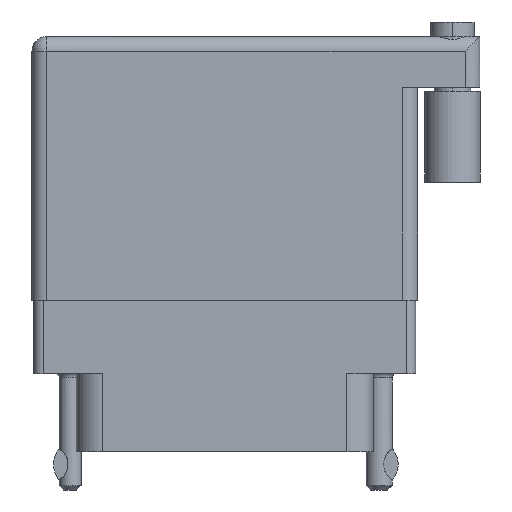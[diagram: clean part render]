
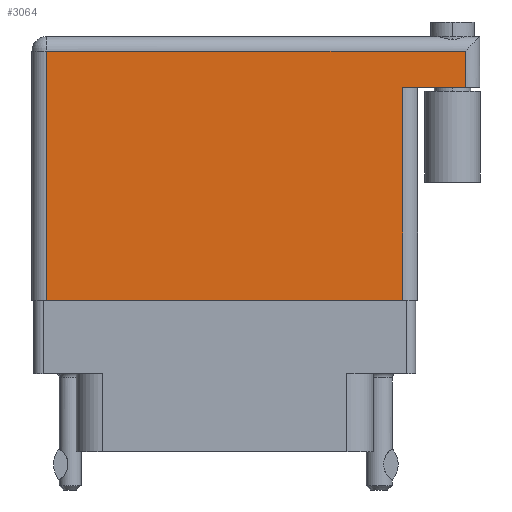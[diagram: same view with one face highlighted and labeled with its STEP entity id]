
A CAD part, front view. The second image highlights one B-rep face of the part: STEP entity #3064.
In plain terms, the highlighted face is planar.
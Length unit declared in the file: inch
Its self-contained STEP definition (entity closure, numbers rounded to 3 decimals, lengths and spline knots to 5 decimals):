
#258 = DIRECTION ( 'NONE',  ( -1., 0., 0. ) ) ;
#670 = EDGE_CURVE ( 'NONE', #27080, #21208, #31366, .T. ) ;
#1006 = ORIENTED_EDGE ( 'NONE', *, *, #4746, .F. ) ;
#1188 = DIRECTION ( 'NONE',  ( 0., 1., 0. ) ) ;
#1465 = CARTESIAN_POINT ( 'NONE',  ( 1.275, 0.731, 0. ) ) ;
#1528 = VERTEX_POINT ( 'NONE', #18580 ) ;
#3013 = LINE ( 'NONE', #14241, #13957 ) ;
#3064 = ADVANCED_FACE ( 'NONE', ( #22866 ), #33910, .F. ) ;
#3598 = VECTOR ( 'NONE', #20691, 39.37008 ) ;
#4746 = EDGE_CURVE ( 'NONE', #9153, #1528, #7953, .T. ) ;
#5846 = EDGE_CURVE ( 'NONE', #21208, #1528, #31854, .T. ) ;
#7746 = EDGE_CURVE ( 'NONE', #24611, #27080, #3013, .T. ) ;
#7953 = LINE ( 'NONE', #18998, #23412 ) ;
#8746 = DIRECTION ( 'NONE',  ( 0., 0., -1. ) ) ;
#8852 = CARTESIAN_POINT ( 'NONE',  ( 0.05, 0.856, 0. ) ) ;
#9110 = CARTESIAN_POINT ( 'NONE',  ( 0., 0.906, 0. ) ) ;
#9153 = VERTEX_POINT ( 'NONE', #26653 ) ;
#11836 = VECTOR ( 'NONE', #1188, 39.37008 ) ;
#12308 = EDGE_CURVE ( 'NONE', #30408, #24611, #19021, .T. ) ;
#13046 = DIRECTION ( 'NONE',  ( 0., 1., 0. ) ) ;
#13957 = VECTOR ( 'NONE', #33417, 39.37008 ) ;
#14241 = CARTESIAN_POINT ( 'NONE',  ( 0.05, 0., 0. ) ) ;
#17090 = EDGE_LOOP ( 'NONE', ( #31367, #17917, #1006, #24808, #35227, #31165 ) ) ;
#17650 = CARTESIAN_POINT ( 'NONE',  ( 0., 0., 0. ) ) ;
#17917 = ORIENTED_EDGE ( 'NONE', *, *, #5846, .T. ) ;
#18580 = CARTESIAN_POINT ( 'NONE',  ( 1.275, 0.731, 0. ) ) ;
#18998 = CARTESIAN_POINT ( 'NONE',  ( 1.539, 0.731, 0. ) ) ;
#19021 = LINE ( 'NONE', #19378, #25669 ) ;
#19378 = CARTESIAN_POINT ( 'NONE',  ( 0., 0.856, 0. ) ) ;
#20565 = VECTOR ( 'NONE', #13046, 39.37008 ) ;
#20691 = DIRECTION ( 'NONE',  ( 1., 0., 0. ) ) ;
#21208 = VERTEX_POINT ( 'NONE', #22982 ) ;
#22262 = CARTESIAN_POINT ( 'NONE',  ( 0.05, 0., 0. ) ) ;
#22857 = CARTESIAN_POINT ( 'NONE',  ( 1.489, 0.856, 0. ) ) ;
#22866 = FACE_OUTER_BOUND ( 'NONE', #17090, .T. ) ;
#22982 = CARTESIAN_POINT ( 'NONE',  ( 1.275, 0., 0. ) ) ;
#23412 = VECTOR ( 'NONE', #26939, 39.37008 ) ;
#24611 = VERTEX_POINT ( 'NONE', #8852 ) ;
#24808 = ORIENTED_EDGE ( 'NONE', *, *, #29060, .T. ) ;
#25422 = CARTESIAN_POINT ( 'NONE',  ( 1.489, 0.906, 0. ) ) ;
#25669 = VECTOR ( 'NONE', #27666, 39.37008 ) ;
#26653 = CARTESIAN_POINT ( 'NONE',  ( 1.489, 0.731, 0. ) ) ;
#26939 = DIRECTION ( 'NONE',  ( -1., 0., 0. ) ) ;
#27080 = VERTEX_POINT ( 'NONE', #22262 ) ;
#27666 = DIRECTION ( 'NONE',  ( -1., 0., 0. ) ) ;
#28705 = LINE ( 'NONE', #25422, #11836 ) ;
#29060 = EDGE_CURVE ( 'NONE', #9153, #30408, #28705, .T. ) ;
#30408 = VERTEX_POINT ( 'NONE', #22857 ) ;
#31165 = ORIENTED_EDGE ( 'NONE', *, *, #7746, .T. ) ;
#31366 = LINE ( 'NONE', #17650, #3598 ) ;
#31367 = ORIENTED_EDGE ( 'NONE', *, *, #670, .T. ) ;
#31854 = LINE ( 'NONE', #1465, #20565 ) ;
#33417 = DIRECTION ( 'NONE',  ( 0., -1., 0. ) ) ;
#33910 = PLANE ( 'NONE',  #34505 ) ;
#34505 = AXIS2_PLACEMENT_3D ( 'NONE', #9110, #8746, #258 ) ;
#35227 = ORIENTED_EDGE ( 'NONE', *, *, #12308, .T. ) ;
